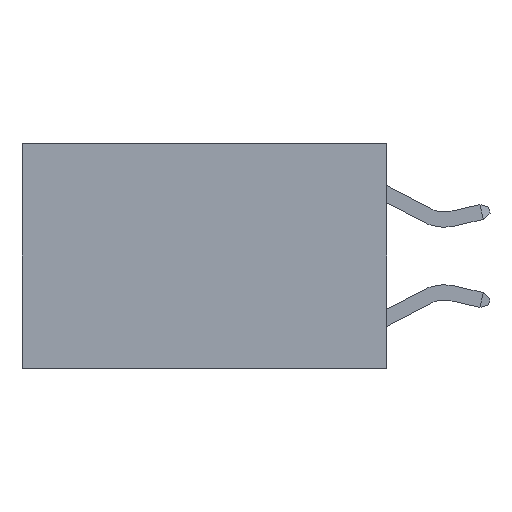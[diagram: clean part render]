
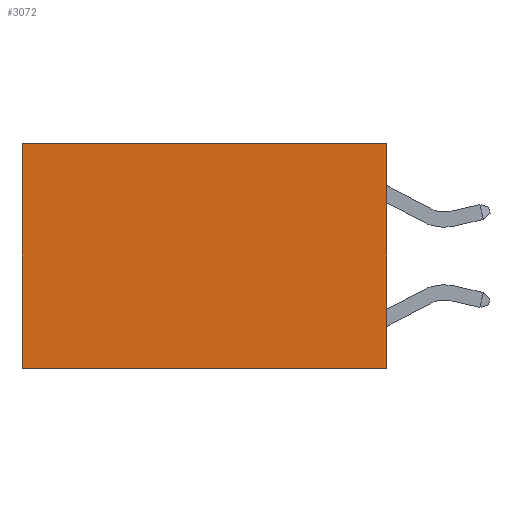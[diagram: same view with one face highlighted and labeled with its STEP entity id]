
A CAD part, left-side view. The second image highlights one B-rep face of the part: STEP entity #3072.
In plain terms, the highlighted planar face has unit normal (-1, 0, 0).
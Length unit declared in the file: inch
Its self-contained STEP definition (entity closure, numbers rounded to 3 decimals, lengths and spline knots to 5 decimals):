
#353 = EDGE_LOOP ( 'NONE', ( #10281, #6938, #13833, #3628 ) ) ;
#1296 = EDGE_CURVE ( 'NONE', #5164, #9218, #12819, .T. ) ;
#1517 = LINE ( 'NONE', #14188, #4822 ) ;
#2430 = VERTEX_POINT ( 'NONE', #2527 ) ;
#2527 = CARTESIAN_POINT ( 'NONE',  ( 0.2625, 0., 0. ) ) ;
#2766 = DIRECTION ( 'NONE',  ( 0., 0., -1. ) ) ;
#2967 = AXIS2_PLACEMENT_3D ( 'NONE', #3193, #14290, #7670 ) ;
#3072 = ADVANCED_FACE ( 'NONE', ( #13773 ), #6539, .F. ) ;
#3193 = CARTESIAN_POINT ( 'NONE',  ( 0.2625, 0., 0. ) ) ;
#3628 = ORIENTED_EDGE ( 'NONE', *, *, #8727, .T. ) ;
#4313 = DIRECTION ( 'NONE',  ( 0., 1., 0. ) ) ;
#4485 = VERTEX_POINT ( 'NONE', #9120 ) ;
#4758 = DIRECTION ( 'NONE',  ( 0., 1., 0. ) ) ;
#4822 = VECTOR ( 'NONE', #6443, 39.37008 ) ;
#5164 = VERTEX_POINT ( 'NONE', #11334 ) ;
#5875 = CARTESIAN_POINT ( 'NONE',  ( 0.2625, 0.6, -0.37 ) ) ;
#6132 = VECTOR ( 'NONE', #2766, 39.37008 ) ;
#6443 = DIRECTION ( 'NONE',  ( 0., 0., -1. ) ) ;
#6539 = PLANE ( 'NONE',  #2967 ) ;
#6938 = ORIENTED_EDGE ( 'NONE', *, *, #1296, .F. ) ;
#7203 = CARTESIAN_POINT ( 'NONE',  ( 0.2625, 0.6, 0. ) ) ;
#7670 = DIRECTION ( 'NONE',  ( 0., 0., -1. ) ) ;
#8404 = EDGE_CURVE ( 'NONE', #2430, #5164, #1517, .T. ) ;
#8727 = EDGE_CURVE ( 'NONE', #2430, #4485, #8815, .T. ) ;
#8815 = LINE ( 'NONE', #11419, #14357 ) ;
#9078 = LINE ( 'NONE', #7203, #6132 ) ;
#9120 = CARTESIAN_POINT ( 'NONE',  ( 0.2625, 0.6, 0. ) ) ;
#9218 = VERTEX_POINT ( 'NONE', #5875 ) ;
#9997 = CARTESIAN_POINT ( 'NONE',  ( 0.2625, 0., -0.37 ) ) ;
#10281 = ORIENTED_EDGE ( 'NONE', *, *, #11902, .T. ) ;
#11334 = CARTESIAN_POINT ( 'NONE',  ( 0.2625, 0., -0.37 ) ) ;
#11419 = CARTESIAN_POINT ( 'NONE',  ( 0.2625, 0., 0. ) ) ;
#11902 = EDGE_CURVE ( 'NONE', #4485, #9218, #9078, .T. ) ;
#12495 = VECTOR ( 'NONE', #4313, 39.37008 ) ;
#12819 = LINE ( 'NONE', #9997, #12495 ) ;
#13773 = FACE_OUTER_BOUND ( 'NONE', #353, .T. ) ;
#13833 = ORIENTED_EDGE ( 'NONE', *, *, #8404, .F. ) ;
#14188 = CARTESIAN_POINT ( 'NONE',  ( 0.2625, 0., 0. ) ) ;
#14290 = DIRECTION ( 'NONE',  ( 1., 0., 0. ) ) ;
#14357 = VECTOR ( 'NONE', #4758, 39.37008 ) ;
